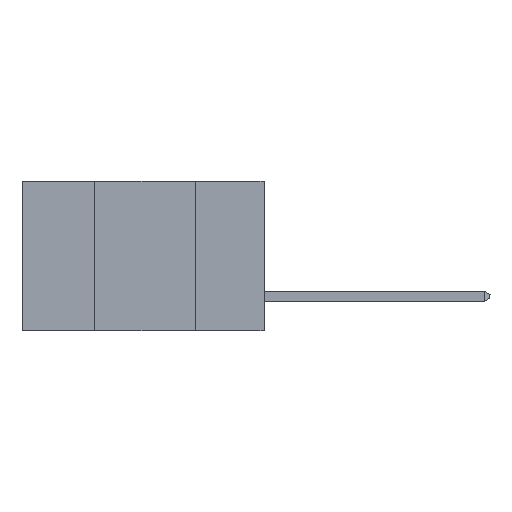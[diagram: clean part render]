
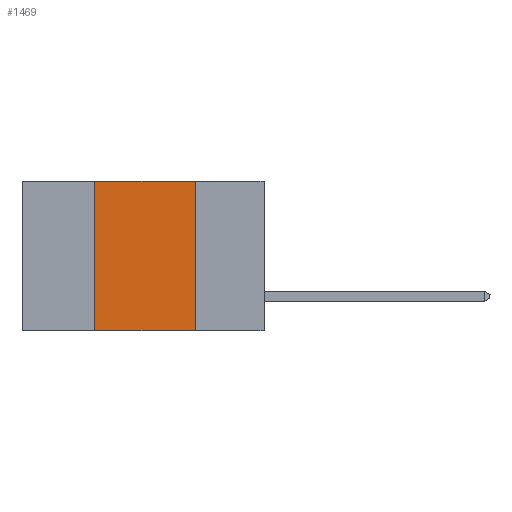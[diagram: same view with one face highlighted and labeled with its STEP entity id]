
A CAD part, left-side view. The second image highlights one B-rep face of the part: STEP entity #1469.
In plain terms, the highlighted planar face has unit normal (-1, 0, 0).
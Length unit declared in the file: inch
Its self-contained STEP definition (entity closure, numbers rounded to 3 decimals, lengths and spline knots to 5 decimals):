
#211 = CARTESIAN_POINT ( 'NONE',  ( 0., 0.17, 0. ) ) ;
#1036 = DIRECTION ( 'NONE',  ( 1., 0., 0. ) ) ;
#1044 = VERTEX_POINT ( 'NONE', #10198 ) ;
#1429 = VERTEX_POINT ( 'NONE', #211 ) ;
#1469 = ADVANCED_FACE ( 'NONE', ( #3874 ), #2934, .F. ) ;
#1672 = ORIENTED_EDGE ( 'NONE', *, *, #5166, .F. ) ;
#1702 = DIRECTION ( 'NONE',  ( 0., -1., 0. ) ) ;
#1907 = CARTESIAN_POINT ( 'NONE',  ( 0., 0.6, -0.37 ) ) ;
#2934 = PLANE ( 'NONE',  #3861 ) ;
#3694 = VECTOR ( 'NONE', #1702, 39.37008 ) ;
#3735 = LINE ( 'NONE', #1907, #8381 ) ;
#3861 = AXIS2_PLACEMENT_3D ( 'NONE', #5509, #1036, #10917 ) ;
#3874 = FACE_OUTER_BOUND ( 'NONE', #10984, .T. ) ;
#3952 = CARTESIAN_POINT ( 'NONE',  ( 0., 0.17, -0.37 ) ) ;
#4018 = CARTESIAN_POINT ( 'NONE',  ( 0., 0.17, -0.37 ) ) ;
#4151 = ORIENTED_EDGE ( 'NONE', *, *, #9703, .F. ) ;
#4480 = CARTESIAN_POINT ( 'NONE',  ( 0., 0.6, 0. ) ) ;
#4529 = EDGE_CURVE ( 'NONE', #1044, #9800, #3735, .T. ) ;
#4719 = CARTESIAN_POINT ( 'NONE',  ( 0., 0.42, -0.37 ) ) ;
#4859 = CARTESIAN_POINT ( 'NONE',  ( 0., 0.42, 0. ) ) ;
#5166 = EDGE_CURVE ( 'NONE', #5531, #1429, #11562, .T. ) ;
#5509 = CARTESIAN_POINT ( 'NONE',  ( 0., 0.6, 0. ) ) ;
#5531 = VERTEX_POINT ( 'NONE', #4859 ) ;
#6426 = DIRECTION ( 'NONE',  ( 0., -1., 0. ) ) ;
#6456 = LINE ( 'NONE', #4719, #7481 ) ;
#6512 = DIRECTION ( 'NONE',  ( 0., 0., 1. ) ) ;
#6681 = DIRECTION ( 'NONE',  ( 0., 0., -1. ) ) ;
#6724 = VECTOR ( 'NONE', #6681, 39.37008 ) ;
#7481 = VECTOR ( 'NONE', #6512, 39.37008 ) ;
#8293 = LINE ( 'NONE', #4018, #6724 ) ;
#8381 = VECTOR ( 'NONE', #6426, 39.37008 ) ;
#9171 = ORIENTED_EDGE ( 'NONE', *, *, #9760, .F. ) ;
#9703 = EDGE_CURVE ( 'NONE', #1429, #9800, #8293, .T. ) ;
#9760 = EDGE_CURVE ( 'NONE', #1044, #5531, #6456, .T. ) ;
#9800 = VERTEX_POINT ( 'NONE', #3952 ) ;
#10198 = CARTESIAN_POINT ( 'NONE',  ( 0., 0.42, -0.37 ) ) ;
#10660 = ORIENTED_EDGE ( 'NONE', *, *, #4529, .T. ) ;
#10917 = DIRECTION ( 'NONE',  ( 0., 0., -1. ) ) ;
#10984 = EDGE_LOOP ( 'NONE', ( #4151, #1672, #9171, #10660 ) ) ;
#11562 = LINE ( 'NONE', #4480, #3694 ) ;
